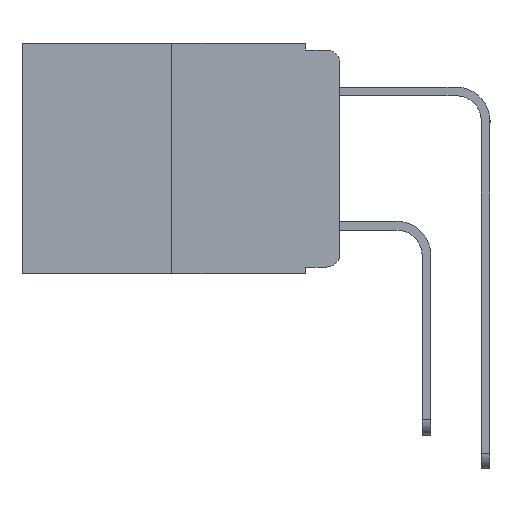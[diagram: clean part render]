
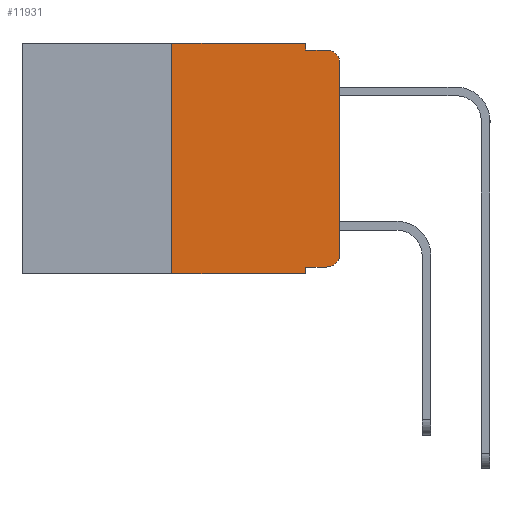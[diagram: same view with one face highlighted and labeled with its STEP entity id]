
A CAD part, left-side view. The second image highlights one B-rep face of the part: STEP entity #11931.
In plain terms, the highlighted planar face has unit normal (-1, 0, 0).
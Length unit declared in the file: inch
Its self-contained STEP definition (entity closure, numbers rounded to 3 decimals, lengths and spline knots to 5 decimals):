
#584 = VERTEX_POINT ( 'NONE', #13696 ) ;
#613 = EDGE_LOOP ( 'NONE', ( #9264, #9657, #12852, #682, #10789, #1111, #4586, #15122, #15507, #2769 ) ) ;
#682 = ORIENTED_EDGE ( 'NONE', *, *, #8009, .F. ) ;
#1111 = ORIENTED_EDGE ( 'NONE', *, *, #6437, .F. ) ;
#1220 = VERTEX_POINT ( 'NONE', #6008 ) ;
#1318 = LINE ( 'NONE', #13195, #7710 ) ;
#1481 = VECTOR ( 'NONE', #13613, 39.37008 ) ;
#1697 = VERTEX_POINT ( 'NONE', #4768 ) ;
#1758 = VECTOR ( 'NONE', #15585, 39.37008 ) ;
#1907 = CARTESIAN_POINT ( 'NONE',  ( 0., 0.051, 0. ) ) ;
#2011 = DIRECTION ( 'NONE',  ( 0., 0., -1. ) ) ;
#2325 = VECTOR ( 'NONE', #7216, 39.37008 ) ;
#2543 = VECTOR ( 'NONE', #12535, 39.37008 ) ;
#2700 = LINE ( 'NONE', #13721, #8642 ) ;
#2745 = CARTESIAN_POINT ( 'NONE',  ( 0., 0.25, -0.343 ) ) ;
#2749 = VERTEX_POINT ( 'NONE', #9233 ) ;
#2769 = ORIENTED_EDGE ( 'NONE', *, *, #3716, .T. ) ;
#2826 = CARTESIAN_POINT ( 'NONE',  ( 0., 0.051, 0. ) ) ;
#3023 = DIRECTION ( 'NONE',  ( 0., 0., -1. ) ) ;
#3120 = AXIS2_PLACEMENT_3D ( 'NONE', #15729, #15879, #15849 ) ;
#3555 = PLANE ( 'NONE',  #7730 ) ;
#3600 = VERTEX_POINT ( 'NONE', #2745 ) ;
#3612 = DIRECTION ( 'NONE',  ( 1., 0., 0. ) ) ;
#3716 = EDGE_CURVE ( 'NONE', #5253, #15773, #14231, .T. ) ;
#3823 = CARTESIAN_POINT ( 'NONE',  ( 0., 0., -0.313 ) ) ;
#3890 = CARTESIAN_POINT ( 'NONE',  ( 0., 0., 0. ) ) ;
#3921 = CARTESIAN_POINT ( 'NONE',  ( 0., 0.25, 0. ) ) ;
#4353 = VECTOR ( 'NONE', #2011, 39.37008 ) ;
#4586 = ORIENTED_EDGE ( 'NONE', *, *, #8648, .T. ) ;
#4768 = CARTESIAN_POINT ( 'NONE',  ( 0., 0.051, -0.01 ) ) ;
#4949 = LINE ( 'NONE', #6296, #1481 ) ;
#5006 = CIRCLE ( 'NONE', #3120, 0.02 ) ;
#5250 = CARTESIAN_POINT ( 'NONE',  ( 0., 0.473, -0.343 ) ) ;
#5253 = VERTEX_POINT ( 'NONE', #13938 ) ;
#5404 = EDGE_CURVE ( 'NONE', #2749, #1220, #5006, .T. ) ;
#5950 = CARTESIAN_POINT ( 'NONE',  ( 0., 0.051, -0.333 ) ) ;
#5966 = LINE ( 'NONE', #3890, #2543 ) ;
#6008 = CARTESIAN_POINT ( 'NONE',  ( 0., 0.02, -0.01 ) ) ;
#6278 = EDGE_CURVE ( 'NONE', #16186, #7250, #14140, .T. ) ;
#6296 = CARTESIAN_POINT ( 'NONE',  ( 0., 0.051, -0.333 ) ) ;
#6370 = LINE ( 'NONE', #8349, #1758 ) ;
#6437 = EDGE_CURVE ( 'NONE', #3600, #584, #15486, .T. ) ;
#6454 = DIRECTION ( 'NONE',  ( 0., 0., -1. ) ) ;
#6723 = DIRECTION ( 'NONE',  ( 0., -1., 0. ) ) ;
#7216 = DIRECTION ( 'NONE',  ( 0., 0., 1. ) ) ;
#7250 = VERTEX_POINT ( 'NONE', #9996 ) ;
#7710 = VECTOR ( 'NONE', #10781, 39.37008 ) ;
#7730 = AXIS2_PLACEMENT_3D ( 'NONE', #15851, #3612, #12258 ) ;
#8009 = EDGE_CURVE ( 'NONE', #14957, #1697, #2700, .T. ) ;
#8182 = AXIS2_PLACEMENT_3D ( 'NONE', #12587, #8737, #3023 ) ;
#8349 = CARTESIAN_POINT ( 'NONE',  ( 0., 0.473, 0. ) ) ;
#8642 = VECTOR ( 'NONE', #6454, 39.37008 ) ;
#8648 = EDGE_CURVE ( 'NONE', #3600, #7250, #10079, .T. ) ;
#8737 = DIRECTION ( 'NONE',  ( -1., 0., 0. ) ) ;
#8863 = FACE_OUTER_BOUND ( 'NONE', #613, .T. ) ;
#9233 = CARTESIAN_POINT ( 'NONE',  ( 0., 0., -0.03 ) ) ;
#9264 = ORIENTED_EDGE ( 'NONE', *, *, #11465, .T. ) ;
#9657 = ORIENTED_EDGE ( 'NONE', *, *, #5404, .T. ) ;
#9722 = VECTOR ( 'NONE', #6723, 39.37008 ) ;
#9996 = CARTESIAN_POINT ( 'NONE',  ( 0., 0.051, -0.343 ) ) ;
#10079 = LINE ( 'NONE', #5250, #9722 ) ;
#10695 = EDGE_CURVE ( 'NONE', #584, #14957, #6370, .T. ) ;
#10781 = DIRECTION ( 'NONE',  ( 0., -1., 0. ) ) ;
#10789 = ORIENTED_EDGE ( 'NONE', *, *, #10695, .F. ) ;
#11187 = EDGE_CURVE ( 'NONE', #1697, #1220, #1318, .T. ) ;
#11465 = EDGE_CURVE ( 'NONE', #15773, #2749, #5966, .T. ) ;
#11931 = ADVANCED_FACE ( 'NONE', ( #8863 ), #3555, .F. ) ;
#12258 = DIRECTION ( 'NONE',  ( 0., 0., -1. ) ) ;
#12535 = DIRECTION ( 'NONE',  ( 0., 0., 1. ) ) ;
#12587 = CARTESIAN_POINT ( 'NONE',  ( 0., 0.02, -0.313 ) ) ;
#12852 = ORIENTED_EDGE ( 'NONE', *, *, #11187, .F. ) ;
#13195 = CARTESIAN_POINT ( 'NONE',  ( 0., 0.051, -0.01 ) ) ;
#13613 = DIRECTION ( 'NONE',  ( 0., -1., 0. ) ) ;
#13696 = CARTESIAN_POINT ( 'NONE',  ( 0., 0.25, 0. ) ) ;
#13721 = CARTESIAN_POINT ( 'NONE',  ( 0., 0.051, 0. ) ) ;
#13938 = CARTESIAN_POINT ( 'NONE',  ( 0., 0.02, -0.333 ) ) ;
#14140 = LINE ( 'NONE', #1907, #4353 ) ;
#14231 = CIRCLE ( 'NONE', #8182, 0.02 ) ;
#14957 = VERTEX_POINT ( 'NONE', #2826 ) ;
#15122 = ORIENTED_EDGE ( 'NONE', *, *, #6278, .F. ) ;
#15152 = EDGE_CURVE ( 'NONE', #16186, #5253, #4949, .T. ) ;
#15486 = LINE ( 'NONE', #3921, #2325 ) ;
#15507 = ORIENTED_EDGE ( 'NONE', *, *, #15152, .T. ) ;
#15585 = DIRECTION ( 'NONE',  ( 0., -1., 0. ) ) ;
#15729 = CARTESIAN_POINT ( 'NONE',  ( 0., 0.02, -0.03 ) ) ;
#15773 = VERTEX_POINT ( 'NONE', #3823 ) ;
#15849 = DIRECTION ( 'NONE',  ( 0., 0., -1. ) ) ;
#15851 = CARTESIAN_POINT ( 'NONE',  ( 0., 0.473, 0. ) ) ;
#15879 = DIRECTION ( 'NONE',  ( -1., 0., 0. ) ) ;
#16186 = VERTEX_POINT ( 'NONE', #5950 ) ;
